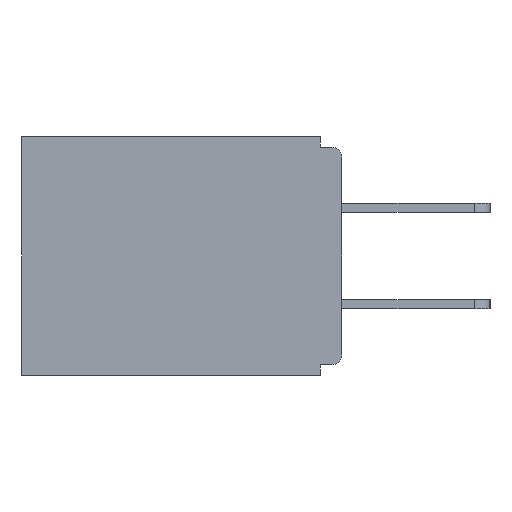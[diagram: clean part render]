
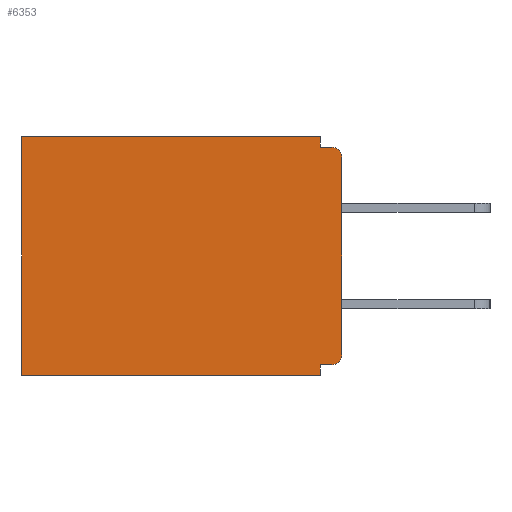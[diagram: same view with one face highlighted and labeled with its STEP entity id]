
A CAD part, left-side view. The second image highlights one B-rep face of the part: STEP entity #6353.
In plain terms, the highlighted planar face has unit normal (-1, 0, 0).
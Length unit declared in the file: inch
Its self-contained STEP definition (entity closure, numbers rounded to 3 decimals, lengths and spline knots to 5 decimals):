
#67 = AXIS2_PLACEMENT_3D ( 'NONE', #2905, #4113, #11768 ) ;
#81 = CARTESIAN_POINT ( 'NONE',  ( 0.298, 0.46, 0. ) ) ;
#131 = VERTEX_POINT ( 'NONE', #10321 ) ;
#608 = CARTESIAN_POINT ( 'NONE',  ( 0.298, 0.015, -0.328 ) ) ;
#830 = ORIENTED_EDGE ( 'NONE', *, *, #3250, .F. ) ;
#857 = LINE ( 'NONE', #5810, #4895 ) ;
#883 = DIRECTION ( 'NONE',  ( 0., 0., -1. ) ) ;
#1198 = CARTESIAN_POINT ( 'NONE',  ( 0.298, 0.031, -0.328 ) ) ;
#1320 = EDGE_CURVE ( 'NONE', #8923, #3781, #2385, .T. ) ;
#1361 = DIRECTION ( 'NONE',  ( 0., 1., 0. ) ) ;
#1457 = VERTEX_POINT ( 'NONE', #1198 ) ;
#1561 = CARTESIAN_POINT ( 'NONE',  ( 0.298, 0.015, -0.313 ) ) ;
#1614 = LINE ( 'NONE', #1732, #11646 ) ;
#1732 = CARTESIAN_POINT ( 'NONE',  ( 0.298, 0.46, 0. ) ) ;
#1755 = CIRCLE ( 'NONE', #9538, 0.015 ) ;
#1925 = PLANE ( 'NONE',  #67 ) ;
#1947 = CARTESIAN_POINT ( 'NONE',  ( 0.298, 0.015, -0.03 ) ) ;
#2248 = VECTOR ( 'NONE', #6185, 39.37008 ) ;
#2262 = ORIENTED_EDGE ( 'NONE', *, *, #11025, .F. ) ;
#2264 = FACE_OUTER_BOUND ( 'NONE', #11159, .T. ) ;
#2385 = CIRCLE ( 'NONE', #8494, 0.015 ) ;
#2443 = EDGE_CURVE ( 'NONE', #12339, #4197, #1614, .T. ) ;
#2561 = VERTEX_POINT ( 'NONE', #8721 ) ;
#2680 = CARTESIAN_POINT ( 'NONE',  ( 0.298, 0., -0.03 ) ) ;
#2905 = CARTESIAN_POINT ( 'NONE',  ( 0.298, 0., 0. ) ) ;
#2929 = DIRECTION ( 'NONE',  ( -1., 0., 0. ) ) ;
#2946 = EDGE_CURVE ( 'NONE', #12005, #3946, #1755, .T. ) ;
#3071 = ORIENTED_EDGE ( 'NONE', *, *, #2443, .T. ) ;
#3087 = VECTOR ( 'NONE', #11957, 39.37008 ) ;
#3250 = EDGE_CURVE ( 'NONE', #6356, #4197, #5825, .T. ) ;
#3781 = VERTEX_POINT ( 'NONE', #12359 ) ;
#3901 = DIRECTION ( 'NONE',  ( 0., 1., 0. ) ) ;
#3946 = VERTEX_POINT ( 'NONE', #5053 ) ;
#4113 = DIRECTION ( 'NONE',  ( 1., 0., 0. ) ) ;
#4197 = VERTEX_POINT ( 'NONE', #5958 ) ;
#4207 = ORIENTED_EDGE ( 'NONE', *, *, #2946, .T. ) ;
#4431 = LINE ( 'NONE', #12038, #3087 ) ;
#4895 = VECTOR ( 'NONE', #3901, 39.37008 ) ;
#5019 = ORIENTED_EDGE ( 'NONE', *, *, #9539, .F. ) ;
#5053 = CARTESIAN_POINT ( 'NONE',  ( 0.298, 0.015, -0.015 ) ) ;
#5105 = CARTESIAN_POINT ( 'NONE',  ( 0.298, 0., 0. ) ) ;
#5305 = CARTESIAN_POINT ( 'NONE',  ( 0.298, 0., -0.343 ) ) ;
#5376 = ORIENTED_EDGE ( 'NONE', *, *, #1320, .T. ) ;
#5575 = LINE ( 'NONE', #7875, #12282 ) ;
#5810 = CARTESIAN_POINT ( 'NONE',  ( 0.298, 0., -0.328 ) ) ;
#5825 = LINE ( 'NONE', #5305, #8958 ) ;
#5958 = CARTESIAN_POINT ( 'NONE',  ( 0.298, 0.46, -0.343 ) ) ;
#6185 = DIRECTION ( 'NONE',  ( 0., -1., 0. ) ) ;
#6341 = LINE ( 'NONE', #5105, #11379 ) ;
#6353 = ADVANCED_FACE ( 'NONE', ( #2264 ), #1925, .F. ) ;
#6356 = VERTEX_POINT ( 'NONE', #7352 ) ;
#6493 = EDGE_CURVE ( 'NONE', #131, #3946, #11254, .T. ) ;
#6574 = ORIENTED_EDGE ( 'NONE', *, *, #6493, .F. ) ;
#6657 = LINE ( 'NONE', #8608, #10761 ) ;
#7352 = CARTESIAN_POINT ( 'NONE',  ( 0.298, 0.031, -0.343 ) ) ;
#7660 = DIRECTION ( 'NONE',  ( 0., 0., -1. ) ) ;
#7812 = DIRECTION ( 'NONE',  ( 0., 1., 0. ) ) ;
#7834 = DIRECTION ( 'NONE',  ( 0., 0., -1. ) ) ;
#7875 = CARTESIAN_POINT ( 'NONE',  ( 0.298, 0.031, -0.343 ) ) ;
#8006 = ORIENTED_EDGE ( 'NONE', *, *, #9948, .F. ) ;
#8007 = CARTESIAN_POINT ( 'NONE',  ( 0.298, 0., -0.015 ) ) ;
#8305 = DIRECTION ( 'NONE',  ( -1., 0., 0. ) ) ;
#8364 = ORIENTED_EDGE ( 'NONE', *, *, #9758, .T. ) ;
#8494 = AXIS2_PLACEMENT_3D ( 'NONE', #1561, #8305, #11148 ) ;
#8608 = CARTESIAN_POINT ( 'NONE',  ( 0.298, 0., 0. ) ) ;
#8721 = CARTESIAN_POINT ( 'NONE',  ( 0.298, 0.031, 0. ) ) ;
#8923 = VERTEX_POINT ( 'NONE', #608 ) ;
#8958 = VECTOR ( 'NONE', #7812, 39.37008 ) ;
#9538 = AXIS2_PLACEMENT_3D ( 'NONE', #1947, #2929, #7660 ) ;
#9539 = EDGE_CURVE ( 'NONE', #12005, #3781, #6657, .T. ) ;
#9758 = EDGE_CURVE ( 'NONE', #2561, #12339, #6341, .T. ) ;
#9850 = DIRECTION ( 'NONE',  ( 0., 0., -1. ) ) ;
#9948 = EDGE_CURVE ( 'NONE', #2561, #131, #5575, .T. ) ;
#10321 = CARTESIAN_POINT ( 'NONE',  ( 0.298, 0.031, -0.015 ) ) ;
#10761 = VECTOR ( 'NONE', #883, 39.37008 ) ;
#11025 = EDGE_CURVE ( 'NONE', #8923, #1457, #857, .T. ) ;
#11148 = DIRECTION ( 'NONE',  ( 0., 0., -1. ) ) ;
#11159 = EDGE_LOOP ( 'NONE', ( #4207, #6574, #8006, #8364, #3071, #830, #12304, #2262, #5376, #5019 ) ) ;
#11254 = LINE ( 'NONE', #8007, #2248 ) ;
#11379 = VECTOR ( 'NONE', #1361, 39.37008 ) ;
#11646 = VECTOR ( 'NONE', #7834, 39.37008 ) ;
#11768 = DIRECTION ( 'NONE',  ( 0., 0., -1. ) ) ;
#11957 = DIRECTION ( 'NONE',  ( 0., 0., -1. ) ) ;
#12005 = VERTEX_POINT ( 'NONE', #2680 ) ;
#12038 = CARTESIAN_POINT ( 'NONE',  ( 0.298, 0.031, -0.343 ) ) ;
#12170 = EDGE_CURVE ( 'NONE', #1457, #6356, #4431, .T. ) ;
#12282 = VECTOR ( 'NONE', #9850, 39.37008 ) ;
#12304 = ORIENTED_EDGE ( 'NONE', *, *, #12170, .F. ) ;
#12339 = VERTEX_POINT ( 'NONE', #81 ) ;
#12359 = CARTESIAN_POINT ( 'NONE',  ( 0.298, 0., -0.313 ) ) ;
